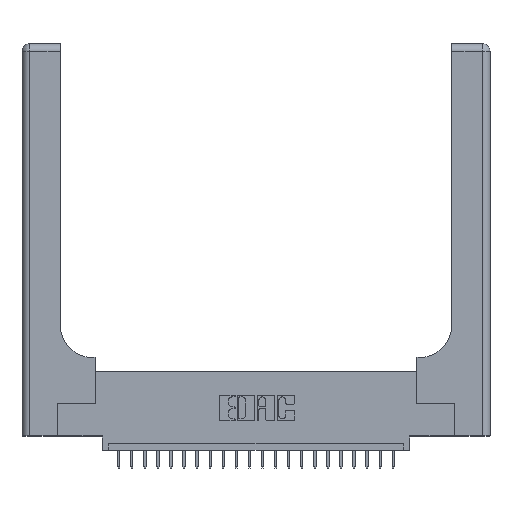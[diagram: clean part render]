
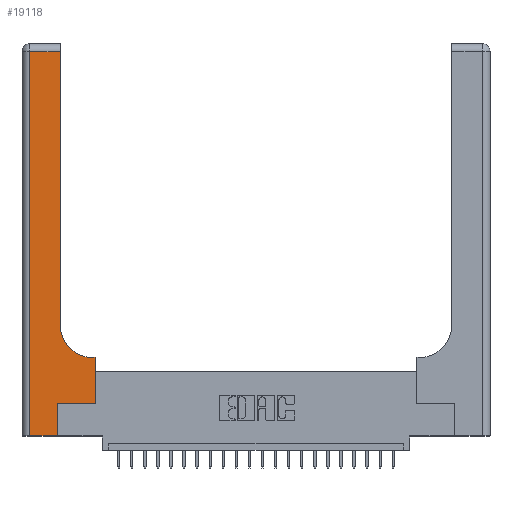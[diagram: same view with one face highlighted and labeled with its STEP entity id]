
A CAD part, top view. The second image highlights one B-rep face of the part: STEP entity #19118.
In plain terms, the highlighted planar face has unit normal (0, 0, 1).
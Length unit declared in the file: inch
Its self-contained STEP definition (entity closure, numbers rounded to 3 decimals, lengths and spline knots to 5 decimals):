
#57 = CARTESIAN_POINT ( 'NONE',  ( 0.2915, 2.94, 0.37 ) ) ;
#155 = DIRECTION ( 'NONE',  ( 0., 1., 0. ) ) ;
#268 = EDGE_CURVE ( 'NONE', #15384, #3565, #13367, .T. ) ;
#469 = CARTESIAN_POINT ( 'NONE',  ( 0.2915, 3., 0.37 ) ) ;
#647 = EDGE_CURVE ( 'NONE', #16410, #7841, #4300, .T. ) ;
#731 = DIRECTION ( 'NONE',  ( 0., 0., -1. ) ) ;
#1494 = DIRECTION ( 'NONE',  ( 0., -1., 0. ) ) ;
#1982 = ORIENTED_EDGE ( 'NONE', *, *, #19836, .T. ) ;
#2495 = VECTOR ( 'NONE', #10964, 39.37008 ) ;
#3565 = VERTEX_POINT ( 'NONE', #8316 ) ;
#3659 = CARTESIAN_POINT ( 'NONE',  ( 0.269, 0., 0.37 ) ) ;
#4300 = LINE ( 'NONE', #469, #8004 ) ;
#4316 = DIRECTION ( 'NONE',  ( -1., 0., 0. ) ) ;
#4564 = CARTESIAN_POINT ( 'NONE',  ( 0.5415, 0.85, 0.37 ) ) ;
#5150 = LINE ( 'NONE', #7261, #9648 ) ;
#5270 = CARTESIAN_POINT ( 'NONE',  ( 0.06, 2.94, 0.37 ) ) ;
#5392 = ORIENTED_EDGE ( 'NONE', *, *, #6234, .T. ) ;
#5510 = CARTESIAN_POINT ( 'NONE',  ( 0.06, 0., 0.37 ) ) ;
#5597 = VECTOR ( 'NONE', #155, 39.37008 ) ;
#6234 = EDGE_CURVE ( 'NONE', #7841, #13242, #6591, .T. ) ;
#6549 = FACE_OUTER_BOUND ( 'NONE', #16152, .T. ) ;
#6591 = LINE ( 'NONE', #10689, #22545 ) ;
#6640 = CARTESIAN_POINT ( 'NONE',  ( 0.5415, 0.6, 0.37 ) ) ;
#6937 = LINE ( 'NONE', #20819, #16544 ) ;
#7261 = CARTESIAN_POINT ( 'NONE',  ( 0.269, 0.25, 0.37 ) ) ;
#7578 = ORIENTED_EDGE ( 'NONE', *, *, #23702, .T. ) ;
#7841 = VERTEX_POINT ( 'NONE', #57 ) ;
#8004 = VECTOR ( 'NONE', #19063, 39.37008 ) ;
#8316 = CARTESIAN_POINT ( 'NONE',  ( 0.5585, 0.6, 0.37 ) ) ;
#8876 = CIRCLE ( 'NONE', #10049, 0.25 ) ;
#9008 = VERTEX_POINT ( 'NONE', #6640 ) ;
#9648 = VECTOR ( 'NONE', #14791, 39.37008 ) ;
#10049 = AXIS2_PLACEMENT_3D ( 'NONE', #4564, #731, #12039 ) ;
#10648 = EDGE_CURVE ( 'NONE', #23318, #16717, #20765, .T. ) ;
#10689 = CARTESIAN_POINT ( 'NONE',  ( 0., 2.94, 0.37 ) ) ;
#10964 = DIRECTION ( 'NONE',  ( 1., 0., 0. ) ) ;
#12039 = DIRECTION ( 'NONE',  ( 1., 0., 0. ) ) ;
#12679 = PLANE ( 'NONE',  #22483 ) ;
#12707 = CARTESIAN_POINT ( 'NONE',  ( 0.2915, 0.85, 0.37 ) ) ;
#13148 = EDGE_CURVE ( 'NONE', #3565, #9008, #21437, .T. ) ;
#13242 = VERTEX_POINT ( 'NONE', #5270 ) ;
#13367 = LINE ( 'NONE', #21106, #5597 ) ;
#13470 = CARTESIAN_POINT ( 'NONE',  ( 0., 0., 0.37 ) ) ;
#14185 = DIRECTION ( 'NONE',  ( -1., 0., 0. ) ) ;
#14791 = DIRECTION ( 'NONE',  ( 1., 0., 0. ) ) ;
#15384 = VERTEX_POINT ( 'NONE', #20970 ) ;
#15388 = CARTESIAN_POINT ( 'NONE',  ( 0.269, 0., 0.37 ) ) ;
#15923 = DIRECTION ( 'NONE',  ( 0., 0., -1. ) ) ;
#16152 = EDGE_LOOP ( 'NONE', ( #18208, #5392, #7578, #1982, #18002, #20208, #17695, #22606, #23445 ) ) ;
#16410 = VERTEX_POINT ( 'NONE', #12707 ) ;
#16544 = VECTOR ( 'NONE', #1494, 39.37008 ) ;
#16717 = VERTEX_POINT ( 'NONE', #21687 ) ;
#16887 = DIRECTION ( 'NONE',  ( 0., 1., 0. ) ) ;
#17695 = ORIENTED_EDGE ( 'NONE', *, *, #268, .T. ) ;
#18002 = ORIENTED_EDGE ( 'NONE', *, *, #10648, .T. ) ;
#18208 = ORIENTED_EDGE ( 'NONE', *, *, #647, .T. ) ;
#18328 = VECTOR ( 'NONE', #16887, 39.37008 ) ;
#18717 = LINE ( 'NONE', #13470, #2495 ) ;
#19063 = DIRECTION ( 'NONE',  ( 0., 1., 0. ) ) ;
#19118 = ADVANCED_FACE ( 'NONE', ( #6549 ), #12679, .F. ) ;
#19815 = CARTESIAN_POINT ( 'NONE',  ( 0.2915, 0.6, 0.37 ) ) ;
#19836 = EDGE_CURVE ( 'NONE', #22334, #23318, #18717, .T. ) ;
#19946 = CARTESIAN_POINT ( 'NONE',  ( 0., 3., 0.37 ) ) ;
#20208 = ORIENTED_EDGE ( 'NONE', *, *, #21361, .T. ) ;
#20765 = LINE ( 'NONE', #3659, #18328 ) ;
#20819 = CARTESIAN_POINT ( 'NONE',  ( 0.06, 3., 0.37 ) ) ;
#20970 = CARTESIAN_POINT ( 'NONE',  ( 0.5585, 0.25, 0.37 ) ) ;
#21106 = CARTESIAN_POINT ( 'NONE',  ( 0.5585, 0.25, 0.37 ) ) ;
#21172 = EDGE_CURVE ( 'NONE', #9008, #16410, #8876, .T. ) ;
#21361 = EDGE_CURVE ( 'NONE', #16717, #15384, #5150, .T. ) ;
#21437 = LINE ( 'NONE', #19815, #21547 ) ;
#21547 = VECTOR ( 'NONE', #4316, 39.37008 ) ;
#21687 = CARTESIAN_POINT ( 'NONE',  ( 0.269, 0.25, 0.37 ) ) ;
#21725 = DIRECTION ( 'NONE',  ( -1., 0., 0. ) ) ;
#22334 = VERTEX_POINT ( 'NONE', #5510 ) ;
#22483 = AXIS2_PLACEMENT_3D ( 'NONE', #19946, #15923, #14185 ) ;
#22545 = VECTOR ( 'NONE', #21725, 39.37008 ) ;
#22606 = ORIENTED_EDGE ( 'NONE', *, *, #13148, .T. ) ;
#23318 = VERTEX_POINT ( 'NONE', #15388 ) ;
#23445 = ORIENTED_EDGE ( 'NONE', *, *, #21172, .T. ) ;
#23702 = EDGE_CURVE ( 'NONE', #13242, #22334, #6937, .T. ) ;
